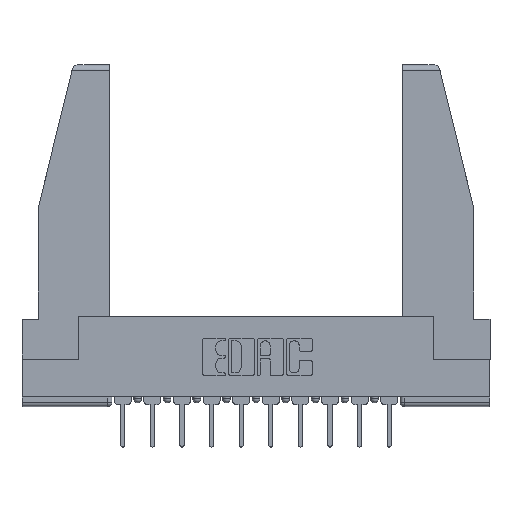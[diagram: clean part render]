
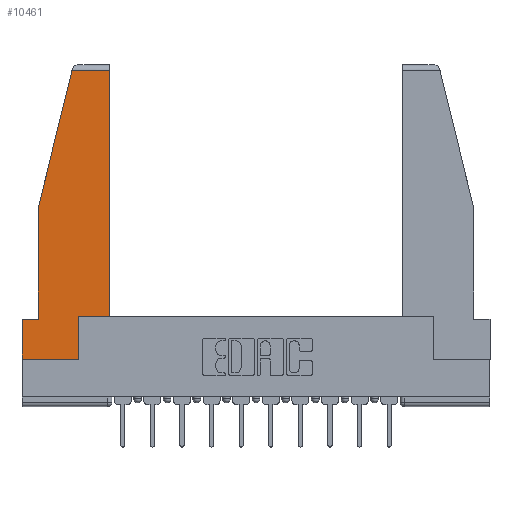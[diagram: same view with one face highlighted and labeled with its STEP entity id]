
A CAD part, top view. The second image highlights one B-rep face of the part: STEP entity #10461.
In plain terms, the highlighted planar face has unit normal (0, 0, 1).
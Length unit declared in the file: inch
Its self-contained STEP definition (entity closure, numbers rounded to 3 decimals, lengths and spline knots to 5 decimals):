
#149 = LINE ( 'NONE', #11712, #13606 ) ;
#546 = CARTESIAN_POINT ( 'NONE',  ( 0.461, 0.223, 0. ) ) ;
#817 = VERTEX_POINT ( 'NONE', #5091 ) ;
#1188 = DIRECTION ( 'NONE',  ( 0., 1., 0. ) ) ;
#1256 = PLANE ( 'NONE',  #4810 ) ;
#1713 = DIRECTION ( 'NONE',  ( 0., -1., 0. ) ) ;
#1874 = VECTOR ( 'NONE', #6818, 39.37008 ) ;
#2174 = ORIENTED_EDGE ( 'NONE', *, *, #3675, .T. ) ;
#2528 = DIRECTION ( 'NONE',  ( 0., 0., 1. ) ) ;
#2706 = ORIENTED_EDGE ( 'NONE', *, *, #6292, .T. ) ;
#2761 = VECTOR ( 'NONE', #9563, 39.37008 ) ;
#2847 = LINE ( 'NONE', #4184, #14944 ) ;
#3207 = LINE ( 'NONE', #7973, #9403 ) ;
#3281 = CARTESIAN_POINT ( 'NONE',  ( 0.271, 1.55, 0. ) ) ;
#3488 = CARTESIAN_POINT ( 'NONE',  ( 0.297, 0., 0. ) ) ;
#3501 = ORIENTED_EDGE ( 'NONE', *, *, #8524, .T. ) ;
#3576 = VERTEX_POINT ( 'NONE', #10399 ) ;
#3675 = EDGE_CURVE ( 'NONE', #8544, #5238, #9044, .T. ) ;
#3697 = CARTESIAN_POINT ( 'NONE',  ( 0.086, 0.8, 0. ) ) ;
#3828 = VERTEX_POINT ( 'NONE', #5078 ) ;
#3875 = CARTESIAN_POINT ( 'NONE',  ( 0., 0., 0. ) ) ;
#4134 = EDGE_CURVE ( 'NONE', #7681, #8977, #5615, .T. ) ;
#4184 = CARTESIAN_POINT ( 'NONE',  ( 0.086, 0.8, 0. ) ) ;
#4420 = VECTOR ( 'NONE', #5029, 39.37008 ) ;
#4430 = EDGE_CURVE ( 'NONE', #13723, #7681, #14452, .T. ) ;
#4732 = VECTOR ( 'NONE', #6482, 39.37008 ) ;
#4770 = LINE ( 'NONE', #3488, #12718 ) ;
#4793 = LINE ( 'NONE', #3875, #2761 ) ;
#4810 = AXIS2_PLACEMENT_3D ( 'NONE', #7213, #2528, #9556 ) ;
#5029 = DIRECTION ( 'NONE',  ( -0.239, -0.971, 0. ) ) ;
#5078 = CARTESIAN_POINT ( 'NONE',  ( 0.086, 0.21, 0. ) ) ;
#5091 = CARTESIAN_POINT ( 'NONE',  ( 0.2636, 1.52, 0. ) ) ;
#5183 = VECTOR ( 'NONE', #1188, 39.37008 ) ;
#5186 = VERTEX_POINT ( 'NONE', #3697 ) ;
#5238 = VERTEX_POINT ( 'NONE', #9607 ) ;
#5295 = ORIENTED_EDGE ( 'NONE', *, *, #9361, .T. ) ;
#5615 = LINE ( 'NONE', #11613, #5183 ) ;
#6079 = DIRECTION ( 'NONE',  ( -1., 0., 0. ) ) ;
#6292 = EDGE_CURVE ( 'NONE', #3576, #13723, #4770, .T. ) ;
#6482 = DIRECTION ( 'NONE',  ( 1., 0., 0. ) ) ;
#6818 = DIRECTION ( 'NONE',  ( 0., -1., 0. ) ) ;
#7213 = CARTESIAN_POINT ( 'NONE',  ( 0., 0., 0. ) ) ;
#7294 = CARTESIAN_POINT ( 'NONE',  ( 0.461, 1.52, 0. ) ) ;
#7681 = VERTEX_POINT ( 'NONE', #546 ) ;
#7973 = CARTESIAN_POINT ( 'NONE',  ( 0., 0.21, 0. ) ) ;
#8524 = EDGE_CURVE ( 'NONE', #3828, #8544, #3207, .T. ) ;
#8544 = VERTEX_POINT ( 'NONE', #14852 ) ;
#8977 = VERTEX_POINT ( 'NONE', #7294 ) ;
#9044 = LINE ( 'NONE', #13643, #1874 ) ;
#9361 = EDGE_CURVE ( 'NONE', #5186, #3828, #2847, .T. ) ;
#9403 = VECTOR ( 'NONE', #10238, 39.37008 ) ;
#9543 = EDGE_LOOP ( 'NONE', ( #9939, #10876, #12309, #5295, #3501, #2174, #10276, #2706, #13845 ) ) ;
#9556 = DIRECTION ( 'NONE',  ( 1., 0., 0. ) ) ;
#9563 = DIRECTION ( 'NONE',  ( 1., 0., 0. ) ) ;
#9607 = CARTESIAN_POINT ( 'NONE',  ( 0., 0., 0. ) ) ;
#9681 = CARTESIAN_POINT ( 'NONE',  ( 0.297, 0.223, 0. ) ) ;
#9939 = ORIENTED_EDGE ( 'NONE', *, *, #4134, .T. ) ;
#10158 = LINE ( 'NONE', #3281, #4420 ) ;
#10238 = DIRECTION ( 'NONE',  ( -1., 0., 0. ) ) ;
#10276 = ORIENTED_EDGE ( 'NONE', *, *, #12480, .T. ) ;
#10399 = CARTESIAN_POINT ( 'NONE',  ( 0.297, 0., 0. ) ) ;
#10460 = DIRECTION ( 'NONE',  ( 0., 1., 0. ) ) ;
#10461 = ADVANCED_FACE ( 'NONE', ( #13946 ), #1256, .T. ) ;
#10559 = CARTESIAN_POINT ( 'NONE',  ( 0.297, 0.223, 0. ) ) ;
#10876 = ORIENTED_EDGE ( 'NONE', *, *, #11463, .T. ) ;
#11463 = EDGE_CURVE ( 'NONE', #8977, #817, #149, .T. ) ;
#11558 = EDGE_CURVE ( 'NONE', #817, #5186, #10158, .T. ) ;
#11613 = CARTESIAN_POINT ( 'NONE',  ( 0.461, 0.223, 0. ) ) ;
#11712 = CARTESIAN_POINT ( 'NONE',  ( 0., 1.52, 0. ) ) ;
#12309 = ORIENTED_EDGE ( 'NONE', *, *, #11558, .T. ) ;
#12480 = EDGE_CURVE ( 'NONE', #5238, #3576, #4793, .T. ) ;
#12718 = VECTOR ( 'NONE', #10460, 39.37008 ) ;
#13606 = VECTOR ( 'NONE', #6079, 39.37008 ) ;
#13643 = CARTESIAN_POINT ( 'NONE',  ( 0., 0.21, 0. ) ) ;
#13723 = VERTEX_POINT ( 'NONE', #10559 ) ;
#13845 = ORIENTED_EDGE ( 'NONE', *, *, #4430, .T. ) ;
#13946 = FACE_OUTER_BOUND ( 'NONE', #9543, .T. ) ;
#14452 = LINE ( 'NONE', #9681, #4732 ) ;
#14852 = CARTESIAN_POINT ( 'NONE',  ( 0., 0.21, 0. ) ) ;
#14944 = VECTOR ( 'NONE', #1713, 39.37008 ) ;
